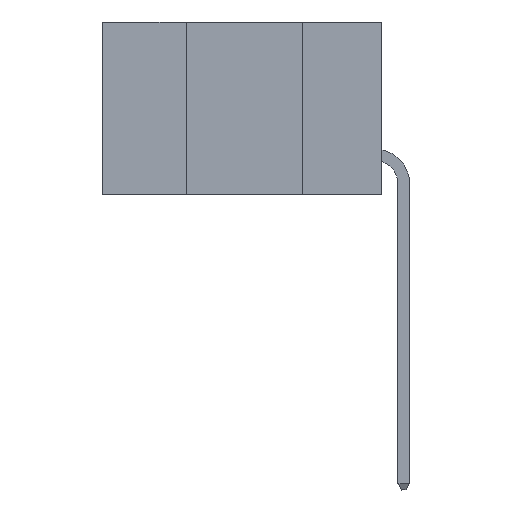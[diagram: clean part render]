
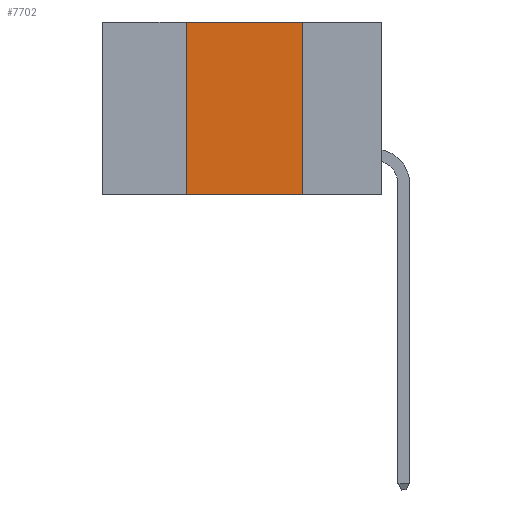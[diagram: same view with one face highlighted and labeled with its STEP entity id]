
A CAD part, left-side view. The second image highlights one B-rep face of the part: STEP entity #7702.
In plain terms, the highlighted planar face has unit normal (-1, 0, 0).
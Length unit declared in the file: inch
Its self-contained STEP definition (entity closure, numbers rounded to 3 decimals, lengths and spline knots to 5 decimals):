
#140 = LINE ( 'NONE', #8404, #21949 ) ;
#215 = DIRECTION ( 'NONE',  ( 0., 0., -1. ) ) ;
#938 = DIRECTION ( 'NONE',  ( 0., 0., 1. ) ) ;
#1251 = DIRECTION ( 'NONE',  ( 0., 0., -1. ) ) ;
#2142 = VECTOR ( 'NONE', #938, 39.37008 ) ;
#2967 = CARTESIAN_POINT ( 'NONE',  ( 0., 0.42, -0.37 ) ) ;
#4388 = EDGE_CURVE ( 'NONE', #20164, #7075, #8575, .T. ) ;
#4991 = EDGE_LOOP ( 'NONE', ( #23710, #5576, #9790, #20687 ) ) ;
#5576 = ORIENTED_EDGE ( 'NONE', *, *, #4388, .F. ) ;
#5678 = FACE_OUTER_BOUND ( 'NONE', #4991, .T. ) ;
#5976 = VERTEX_POINT ( 'NONE', #2967 ) ;
#6478 = CARTESIAN_POINT ( 'NONE',  ( 0., 0.6, 0. ) ) ;
#6909 = AXIS2_PLACEMENT_3D ( 'NONE', #8770, #14735, #1251 ) ;
#7075 = VERTEX_POINT ( 'NONE', #24237 ) ;
#7648 = LINE ( 'NONE', #18896, #19405 ) ;
#7702 = ADVANCED_FACE ( 'NONE', ( #5678 ), #24494, .F. ) ;
#7783 = CARTESIAN_POINT ( 'NONE',  ( 0., 0.17, -0.37 ) ) ;
#8404 = CARTESIAN_POINT ( 'NONE',  ( 0., 0.6, -0.37 ) ) ;
#8465 = DIRECTION ( 'NONE',  ( 0., -1., 0. ) ) ;
#8575 = LINE ( 'NONE', #6478, #14566 ) ;
#8770 = CARTESIAN_POINT ( 'NONE',  ( 0., 0.6, 0. ) ) ;
#9790 = ORIENTED_EDGE ( 'NONE', *, *, #10941, .F. ) ;
#10441 = EDGE_CURVE ( 'NONE', #7075, #19033, #7648, .T. ) ;
#10941 = EDGE_CURVE ( 'NONE', #5976, #20164, #16353, .T. ) ;
#12510 = DIRECTION ( 'NONE',  ( 0., -1., 0. ) ) ;
#12740 = CARTESIAN_POINT ( 'NONE',  ( 0., 0.42, 0. ) ) ;
#14566 = VECTOR ( 'NONE', #8465, 39.37008 ) ;
#14735 = DIRECTION ( 'NONE',  ( 1., 0., 0. ) ) ;
#16353 = LINE ( 'NONE', #12740, #2142 ) ;
#18896 = CARTESIAN_POINT ( 'NONE',  ( 0., 0.17, 0. ) ) ;
#19033 = VERTEX_POINT ( 'NONE', #7783 ) ;
#19405 = VECTOR ( 'NONE', #215, 39.37008 ) ;
#20164 = VERTEX_POINT ( 'NONE', #24622 ) ;
#20687 = ORIENTED_EDGE ( 'NONE', *, *, #21974, .T. ) ;
#21949 = VECTOR ( 'NONE', #12510, 39.37008 ) ;
#21974 = EDGE_CURVE ( 'NONE', #5976, #19033, #140, .T. ) ;
#23710 = ORIENTED_EDGE ( 'NONE', *, *, #10441, .F. ) ;
#24237 = CARTESIAN_POINT ( 'NONE',  ( 0., 0.17, 0. ) ) ;
#24494 = PLANE ( 'NONE',  #6909 ) ;
#24622 = CARTESIAN_POINT ( 'NONE',  ( 0., 0.42, 0. ) ) ;
